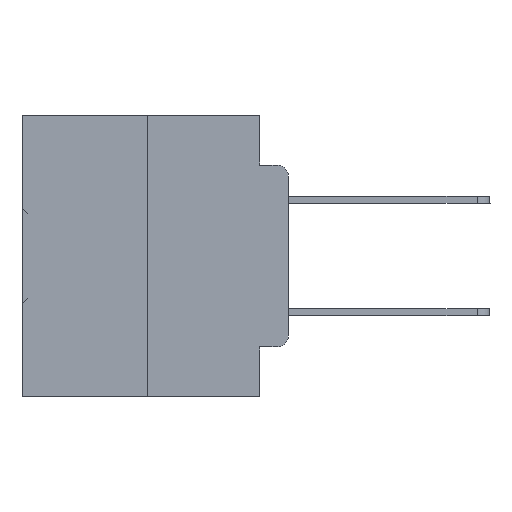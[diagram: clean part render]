
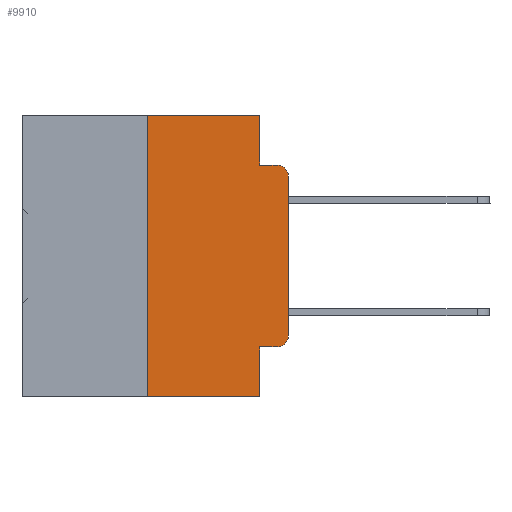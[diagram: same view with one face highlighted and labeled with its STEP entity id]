
A CAD part, left-side view. The second image highlights one B-rep face of the part: STEP entity #9910.
In plain terms, the highlighted planar face has unit normal (-1, 0, 0).
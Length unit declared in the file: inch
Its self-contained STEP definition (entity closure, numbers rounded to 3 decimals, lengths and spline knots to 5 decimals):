
#149 = VERTEX_POINT ( 'NONE', #23281 ) ;
#553 = VERTEX_POINT ( 'NONE', #8058 ) ;
#620 = DIRECTION ( 'NONE',  ( 0., 0., 1. ) ) ;
#1589 = VECTOR ( 'NONE', #17248, 39.37008 ) ;
#1933 = CARTESIAN_POINT ( 'NONE',  ( 0., 0.051, -0.4115 ) ) ;
#1974 = ORIENTED_EDGE ( 'NONE', *, *, #24517, .T. ) ;
#2049 = DIRECTION ( 'NONE',  ( 0., 0., -1. ) ) ;
#2304 = CARTESIAN_POINT ( 'NONE',  ( 0., 0.473, 0. ) ) ;
#2499 = ORIENTED_EDGE ( 'NONE', *, *, #6178, .T. ) ;
#3355 = CARTESIAN_POINT ( 'NONE',  ( 0., 0.051, -0.0885 ) ) ;
#3375 = EDGE_CURVE ( 'NONE', #30938, #21709, #5383, .T. ) ;
#4602 = DIRECTION ( 'NONE',  ( 0., 0., -1. ) ) ;
#5383 = LINE ( 'NONE', #25897, #8168 ) ;
#5742 = CARTESIAN_POINT ( 'NONE',  ( 0., 0.25, -0.5 ) ) ;
#5803 = VECTOR ( 'NONE', #13042, 39.37008 ) ;
#6178 = EDGE_CURVE ( 'NONE', #28802, #553, #21032, .T. ) ;
#6527 = CARTESIAN_POINT ( 'NONE',  ( 0., 0.051, -0.0885 ) ) ;
#8058 = CARTESIAN_POINT ( 'NONE',  ( 0., 0., -0.3915 ) ) ;
#8068 = EDGE_CURVE ( 'NONE', #30938, #28802, #27461, .T. ) ;
#8146 = CARTESIAN_POINT ( 'NONE',  ( 0., 0., -0.1085 ) ) ;
#8168 = VECTOR ( 'NONE', #23051, 39.37008 ) ;
#9462 = LINE ( 'NONE', #26264, #1589 ) ;
#9559 = ORIENTED_EDGE ( 'NONE', *, *, #19044, .F. ) ;
#9910 = ADVANCED_FACE ( 'NONE', ( #18214 ), #16823, .F. ) ;
#10830 = LINE ( 'NONE', #27547, #30863 ) ;
#11573 = CARTESIAN_POINT ( 'NONE',  ( 0., 0.25, 0. ) ) ;
#12136 = ORIENTED_EDGE ( 'NONE', *, *, #24879, .T. ) ;
#12157 = VECTOR ( 'NONE', #17992, 39.37008 ) ;
#12612 = ORIENTED_EDGE ( 'NONE', *, *, #16480, .T. ) ;
#13042 = DIRECTION ( 'NONE',  ( 0., 0., -1. ) ) ;
#13843 = LINE ( 'NONE', #2304, #36656 ) ;
#13937 = ORIENTED_EDGE ( 'NONE', *, *, #16074, .F. ) ;
#15452 = VERTEX_POINT ( 'NONE', #3355 ) ;
#15743 = AXIS2_PLACEMENT_3D ( 'NONE', #28311, #34010, #4602 ) ;
#16074 = EDGE_CURVE ( 'NONE', #25735, #19909, #13843, .T. ) ;
#16480 = EDGE_CURVE ( 'NONE', #30285, #149, #32469, .T. ) ;
#16746 = AXIS2_PLACEMENT_3D ( 'NONE', #35496, #29114, #17653 ) ;
#16823 = PLANE ( 'NONE',  #30574 ) ;
#17088 = DIRECTION ( 'NONE',  ( 0., -1., 0. ) ) ;
#17248 = DIRECTION ( 'NONE',  ( 0., 0., 1. ) ) ;
#17653 = DIRECTION ( 'NONE',  ( 0., 0., -1. ) ) ;
#17992 = DIRECTION ( 'NONE',  ( 0., -1., 0. ) ) ;
#18150 = EDGE_CURVE ( 'NONE', #19909, #15452, #23989, .T. ) ;
#18214 = FACE_OUTER_BOUND ( 'NONE', #38002, .T. ) ;
#19044 = EDGE_CURVE ( 'NONE', #28127, #25735, #9462, .T. ) ;
#19835 = ORIENTED_EDGE ( 'NONE', *, *, #8068, .T. ) ;
#19862 = DIRECTION ( 'NONE',  ( 1., 0., 0. ) ) ;
#19909 = VERTEX_POINT ( 'NONE', #21190 ) ;
#20359 = EDGE_CURVE ( 'NONE', #15452, #149, #22940, .T. ) ;
#20389 = CARTESIAN_POINT ( 'NONE',  ( 0., 0.051, -0.4115 ) ) ;
#21032 = CIRCLE ( 'NONE', #16746, 0.02 ) ;
#21190 = CARTESIAN_POINT ( 'NONE',  ( 0., 0.051, 0. ) ) ;
#21709 = VERTEX_POINT ( 'NONE', #31029 ) ;
#22940 = LINE ( 'NONE', #6527, #12157 ) ;
#22969 = CARTESIAN_POINT ( 'NONE',  ( 0., 0.473, -0.5 ) ) ;
#23051 = DIRECTION ( 'NONE',  ( 0., 0., -1. ) ) ;
#23281 = CARTESIAN_POINT ( 'NONE',  ( 0., 0.02, -0.0885 ) ) ;
#23989 = LINE ( 'NONE', #27535, #5803 ) ;
#24517 = EDGE_CURVE ( 'NONE', #553, #30285, #10830, .T. ) ;
#24879 = EDGE_CURVE ( 'NONE', #28127, #21709, #37779, .T. ) ;
#25735 = VERTEX_POINT ( 'NONE', #11573 ) ;
#25897 = CARTESIAN_POINT ( 'NONE',  ( 0., 0.051, 0. ) ) ;
#26264 = CARTESIAN_POINT ( 'NONE',  ( 0., 0.25, 0. ) ) ;
#27461 = LINE ( 'NONE', #1933, #37187 ) ;
#27535 = CARTESIAN_POINT ( 'NONE',  ( 0., 0.051, 0. ) ) ;
#27547 = CARTESIAN_POINT ( 'NONE',  ( 0., 0., 0. ) ) ;
#28127 = VERTEX_POINT ( 'NONE', #5742 ) ;
#28311 = CARTESIAN_POINT ( 'NONE',  ( 0., 0.02, -0.1085 ) ) ;
#28802 = VERTEX_POINT ( 'NONE', #34968 ) ;
#28961 = DIRECTION ( 'NONE',  ( 0., -1., 0. ) ) ;
#29114 = DIRECTION ( 'NONE',  ( -1., 0., 0. ) ) ;
#30285 = VERTEX_POINT ( 'NONE', #8146 ) ;
#30574 = AXIS2_PLACEMENT_3D ( 'NONE', #37650, #19862, #2049 ) ;
#30863 = VECTOR ( 'NONE', #620, 39.37008 ) ;
#30938 = VERTEX_POINT ( 'NONE', #20389 ) ;
#31029 = CARTESIAN_POINT ( 'NONE',  ( 0., 0.051, -0.5 ) ) ;
#31519 = ORIENTED_EDGE ( 'NONE', *, *, #20359, .F. ) ;
#31923 = ORIENTED_EDGE ( 'NONE', *, *, #18150, .F. ) ;
#32469 = CIRCLE ( 'NONE', #15743, 0.02 ) ;
#34010 = DIRECTION ( 'NONE',  ( -1., 0., 0. ) ) ;
#34547 = VECTOR ( 'NONE', #35027, 39.37008 ) ;
#34968 = CARTESIAN_POINT ( 'NONE',  ( 0., 0.02, -0.4115 ) ) ;
#35027 = DIRECTION ( 'NONE',  ( 0., -1., 0. ) ) ;
#35496 = CARTESIAN_POINT ( 'NONE',  ( 0., 0.02, -0.3915 ) ) ;
#36656 = VECTOR ( 'NONE', #28961, 39.37008 ) ;
#37187 = VECTOR ( 'NONE', #17088, 39.37008 ) ;
#37650 = CARTESIAN_POINT ( 'NONE',  ( 0., 0.473, 0. ) ) ;
#37779 = LINE ( 'NONE', #22969, #34547 ) ;
#37993 = ORIENTED_EDGE ( 'NONE', *, *, #3375, .F. ) ;
#38002 = EDGE_LOOP ( 'NONE', ( #1974, #12612, #31519, #31923, #13937, #9559, #12136, #37993, #19835, #2499 ) ) ;
